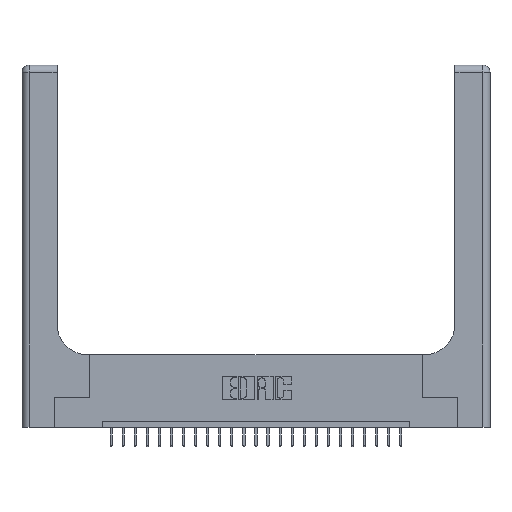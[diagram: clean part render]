
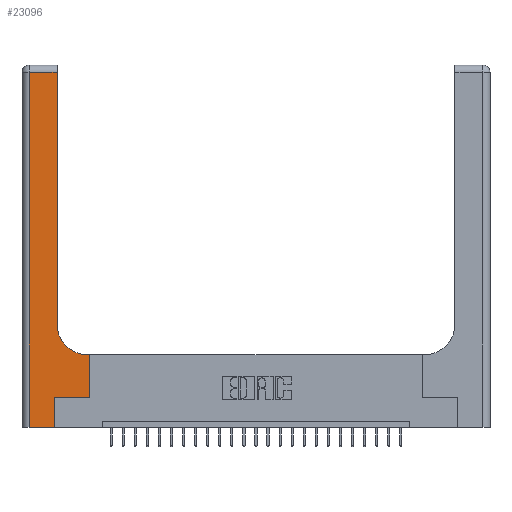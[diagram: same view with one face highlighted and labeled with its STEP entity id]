
A CAD part, top view. The second image highlights one B-rep face of the part: STEP entity #23096.
In plain terms, the highlighted planar face has unit normal (0, 0, 1).
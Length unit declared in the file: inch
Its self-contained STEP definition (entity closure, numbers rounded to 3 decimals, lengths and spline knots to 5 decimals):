
#402 = EDGE_CURVE ( 'NONE', #4289, #14169, #16313, .T. ) ;
#407 = ORIENTED_EDGE ( 'NONE', *, *, #402, .T. ) ;
#649 = EDGE_CURVE ( 'NONE', #10845, #4289, #22627, .T. ) ;
#1237 = DIRECTION ( 'NONE',  ( 0., 1., 0. ) ) ;
#1641 = ORIENTED_EDGE ( 'NONE', *, *, #649, .T. ) ;
#1941 = CARTESIAN_POINT ( 'NONE',  ( 0., 0., 0.37 ) ) ;
#2277 = ORIENTED_EDGE ( 'NONE', *, *, #4225, .T. ) ;
#2327 = AXIS2_PLACEMENT_3D ( 'NONE', #12292, #10284, #22443 ) ;
#2771 = DIRECTION ( 'NONE',  ( 1., 0., 0. ) ) ;
#2842 = DIRECTION ( 'NONE',  ( -1., 0., 0. ) ) ;
#2972 = LINE ( 'NONE', #20966, #4544 ) ;
#4225 = EDGE_CURVE ( 'NONE', #25579, #11612, #15796, .T. ) ;
#4289 = VERTEX_POINT ( 'NONE', #7266 ) ;
#4358 = VECTOR ( 'NONE', #15011, 39.37008 ) ;
#4363 = LINE ( 'NONE', #12827, #11942 ) ;
#4544 = VECTOR ( 'NONE', #2842, 39.37008 ) ;
#4890 = ORIENTED_EDGE ( 'NONE', *, *, #18833, .T. ) ;
#5171 = CARTESIAN_POINT ( 'NONE',  ( 0.5585, 0.25, 0.37 ) ) ;
#5188 = CARTESIAN_POINT ( 'NONE',  ( 0.5585, 0.25, 0.37 ) ) ;
#5663 = CARTESIAN_POINT ( 'NONE',  ( 0.269, 0., 0.37 ) ) ;
#6108 = VECTOR ( 'NONE', #24035, 39.37008 ) ;
#6476 = ORIENTED_EDGE ( 'NONE', *, *, #18353, .T. ) ;
#6970 = VECTOR ( 'NONE', #11376, 39.37008 ) ;
#7266 = CARTESIAN_POINT ( 'NONE',  ( 0.269, 0.25, 0.37 ) ) ;
#7751 = EDGE_CURVE ( 'NONE', #14169, #24446, #25809, .T. ) ;
#8091 = CARTESIAN_POINT ( 'NONE',  ( 0.5585, 0.6, 0.37 ) ) ;
#8223 = VERTEX_POINT ( 'NONE', #10544 ) ;
#8724 = DIRECTION ( 'NONE',  ( 0., 0., -1. ) ) ;
#8779 = EDGE_LOOP ( 'NONE', ( #2277, #4890, #19346, #12360, #1641, #407, #9300, #25135, #6476 ) ) ;
#9156 = CARTESIAN_POINT ( 'NONE',  ( 0.2915, 3., 0.37 ) ) ;
#9300 = ORIENTED_EDGE ( 'NONE', *, *, #7751, .T. ) ;
#9316 = CARTESIAN_POINT ( 'NONE',  ( 0.2915, 0.85, 0.37 ) ) ;
#10195 = CARTESIAN_POINT ( 'NONE',  ( 0.2915, 2.94, 0.37 ) ) ;
#10284 = DIRECTION ( 'NONE',  ( 0., 0., -1. ) ) ;
#10544 = CARTESIAN_POINT ( 'NONE',  ( 0.06, 2.94, 0.37 ) ) ;
#10590 = VERTEX_POINT ( 'NONE', #11469 ) ;
#10623 = PLANE ( 'NONE',  #2327 ) ;
#10845 = VERTEX_POINT ( 'NONE', #17666 ) ;
#10952 = CIRCLE ( 'NONE', #19437, 0.25 ) ;
#11376 = DIRECTION ( 'NONE',  ( -1., 0., 0. ) ) ;
#11448 = CARTESIAN_POINT ( 'NONE',  ( 0.269, 0.25, 0.37 ) ) ;
#11469 = CARTESIAN_POINT ( 'NONE',  ( 0.5415, 0.6, 0.37 ) ) ;
#11612 = VERTEX_POINT ( 'NONE', #10195 ) ;
#11942 = VECTOR ( 'NONE', #14884, 39.37008 ) ;
#12292 = CARTESIAN_POINT ( 'NONE',  ( 0., 3., 0.37 ) ) ;
#12360 = ORIENTED_EDGE ( 'NONE', *, *, #25133, .T. ) ;
#12827 = CARTESIAN_POINT ( 'NONE',  ( 0.06, 3., 0.37 ) ) ;
#12987 = LINE ( 'NONE', #15439, #6970 ) ;
#13823 = DIRECTION ( 'NONE',  ( 0., 1., 0. ) ) ;
#14169 = VERTEX_POINT ( 'NONE', #5188 ) ;
#14351 = VECTOR ( 'NONE', #1237, 39.37008 ) ;
#14884 = DIRECTION ( 'NONE',  ( 0., -1., 0. ) ) ;
#15011 = DIRECTION ( 'NONE',  ( 0., 1., 0. ) ) ;
#15439 = CARTESIAN_POINT ( 'NONE',  ( 0.2915, 0.6, 0.37 ) ) ;
#15796 = LINE ( 'NONE', #9156, #4358 ) ;
#16313 = LINE ( 'NONE', #11448, #20744 ) ;
#16508 = EDGE_CURVE ( 'NONE', #8223, #19171, #4363, .T. ) ;
#17666 = CARTESIAN_POINT ( 'NONE',  ( 0.269, 0., 0.37 ) ) ;
#17744 = DIRECTION ( 'NONE',  ( 1., 0., 0. ) ) ;
#18353 = EDGE_CURVE ( 'NONE', #10590, #25579, #10952, .T. ) ;
#18534 = CARTESIAN_POINT ( 'NONE',  ( 0.06, 0., 0.37 ) ) ;
#18833 = EDGE_CURVE ( 'NONE', #11612, #8223, #2972, .T. ) ;
#19171 = VERTEX_POINT ( 'NONE', #18534 ) ;
#19346 = ORIENTED_EDGE ( 'NONE', *, *, #16508, .T. ) ;
#19437 = AXIS2_PLACEMENT_3D ( 'NONE', #25055, #8724, #2771 ) ;
#20744 = VECTOR ( 'NONE', #17744, 39.37008 ) ;
#20966 = CARTESIAN_POINT ( 'NONE',  ( 0., 2.94, 0.37 ) ) ;
#21129 = EDGE_CURVE ( 'NONE', #24446, #10590, #12987, .T. ) ;
#22443 = DIRECTION ( 'NONE',  ( -1., 0., 0. ) ) ;
#22627 = LINE ( 'NONE', #5663, #23259 ) ;
#23096 = ADVANCED_FACE ( 'NONE', ( #23341 ), #10623, .F. ) ;
#23259 = VECTOR ( 'NONE', #13823, 39.37008 ) ;
#23341 = FACE_OUTER_BOUND ( 'NONE', #8779, .T. ) ;
#24035 = DIRECTION ( 'NONE',  ( 1., 0., 0. ) ) ;
#24446 = VERTEX_POINT ( 'NONE', #8091 ) ;
#24859 = LINE ( 'NONE', #1941, #6108 ) ;
#25055 = CARTESIAN_POINT ( 'NONE',  ( 0.5415, 0.85, 0.37 ) ) ;
#25133 = EDGE_CURVE ( 'NONE', #19171, #10845, #24859, .T. ) ;
#25135 = ORIENTED_EDGE ( 'NONE', *, *, #21129, .T. ) ;
#25579 = VERTEX_POINT ( 'NONE', #9316 ) ;
#25809 = LINE ( 'NONE', #5171, #14351 ) ;
